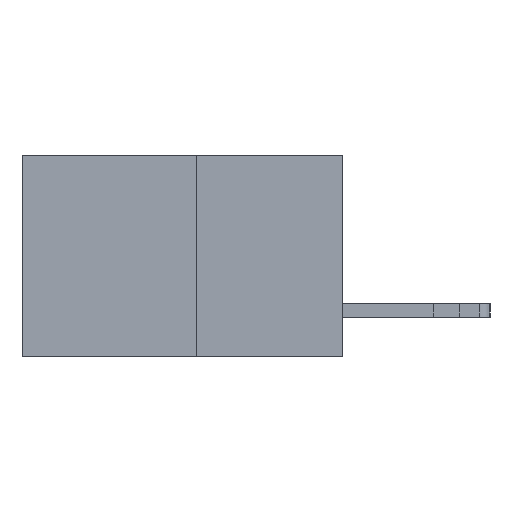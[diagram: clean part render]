
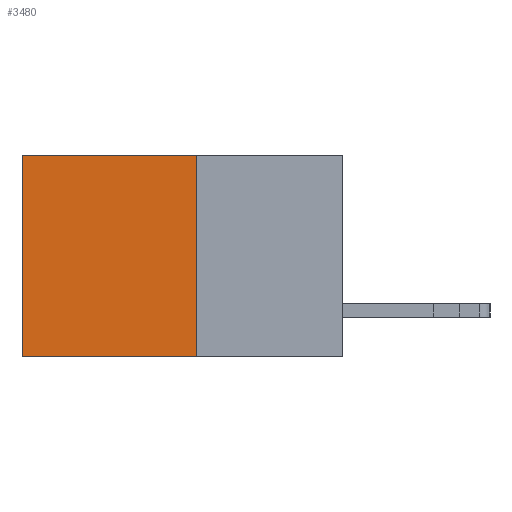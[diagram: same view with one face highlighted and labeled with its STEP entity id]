
A CAD part, left-side view. The second image highlights one B-rep face of the part: STEP entity #3480.
In plain terms, the highlighted planar face has unit normal (-1, 0, 0).
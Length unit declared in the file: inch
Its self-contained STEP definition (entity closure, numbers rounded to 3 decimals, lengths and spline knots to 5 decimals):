
#118 = CARTESIAN_POINT ( 'NONE',  ( 0.277, 0.27, -0.37 ) ) ;
#380 = ORIENTED_EDGE ( 'NONE', *, *, #2233, .T. ) ;
#419 = FACE_OUTER_BOUND ( 'NONE', #9409, .T. ) ;
#595 = DIRECTION ( 'NONE',  ( 0., 0., -1. ) ) ;
#1267 = PLANE ( 'NONE',  #9873 ) ;
#1471 = VECTOR ( 'NONE', #2577, 39.37008 ) ;
#1743 = CARTESIAN_POINT ( 'NONE',  ( 0.277, 0.59, -0.37 ) ) ;
#1765 = DIRECTION ( 'NONE',  ( 1., 0., 0. ) ) ;
#2019 = CARTESIAN_POINT ( 'NONE',  ( 0.277, 0.59, -0.37 ) ) ;
#2101 = DIRECTION ( 'NONE',  ( 0., 0., -1. ) ) ;
#2233 = EDGE_CURVE ( 'NONE', #13475, #8363, #13564, .T. ) ;
#2255 = DIRECTION ( 'NONE',  ( 0., 1., 0. ) ) ;
#2577 = DIRECTION ( 'NONE',  ( 0., 0., -1. ) ) ;
#2587 = CARTESIAN_POINT ( 'NONE',  ( 0.277, 0.27, -0.37 ) ) ;
#2953 = ORIENTED_EDGE ( 'NONE', *, *, #11268, .F. ) ;
#3006 = CARTESIAN_POINT ( 'NONE',  ( 0.277, 0.27, 0. ) ) ;
#3134 = ORIENTED_EDGE ( 'NONE', *, *, #8282, .F. ) ;
#3480 = ADVANCED_FACE ( 'NONE', ( #419 ), #1267, .F. ) ;
#3584 = LINE ( 'NONE', #10866, #10367 ) ;
#3663 = DIRECTION ( 'NONE',  ( 0., 1., 0. ) ) ;
#4414 = CARTESIAN_POINT ( 'NONE',  ( 0.277, 0.59, 0. ) ) ;
#6388 = VERTEX_POINT ( 'NONE', #3006 ) ;
#7128 = VECTOR ( 'NONE', #2255, 39.37008 ) ;
#7946 = LINE ( 'NONE', #2587, #1471 ) ;
#8282 = EDGE_CURVE ( 'NONE', #6388, #15260, #7946, .T. ) ;
#8307 = ORIENTED_EDGE ( 'NONE', *, *, #10029, .T. ) ;
#8363 = VERTEX_POINT ( 'NONE', #1743 ) ;
#9174 = CARTESIAN_POINT ( 'NONE',  ( 0.277, 0.27, -0.37 ) ) ;
#9409 = EDGE_LOOP ( 'NONE', ( #380, #2953, #3134, #8307 ) ) ;
#9873 = AXIS2_PLACEMENT_3D ( 'NONE', #118, #1765, #595 ) ;
#10029 = EDGE_CURVE ( 'NONE', #6388, #13475, #3584, .T. ) ;
#10367 = VECTOR ( 'NONE', #3663, 39.37008 ) ;
#10521 = VECTOR ( 'NONE', #2101, 39.37008 ) ;
#10866 = CARTESIAN_POINT ( 'NONE',  ( 0.277, 0.27, 0. ) ) ;
#11268 = EDGE_CURVE ( 'NONE', #15260, #8363, #13004, .T. ) ;
#12957 = CARTESIAN_POINT ( 'NONE',  ( 0.277, 0.27, -0.37 ) ) ;
#13004 = LINE ( 'NONE', #12957, #7128 ) ;
#13475 = VERTEX_POINT ( 'NONE', #4414 ) ;
#13564 = LINE ( 'NONE', #2019, #10521 ) ;
#15260 = VERTEX_POINT ( 'NONE', #9174 ) ;
